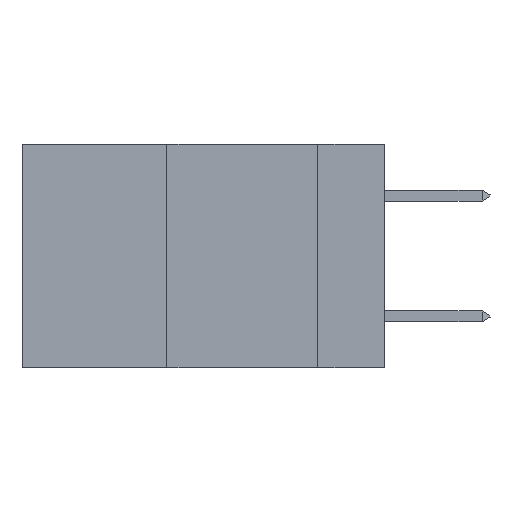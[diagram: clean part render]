
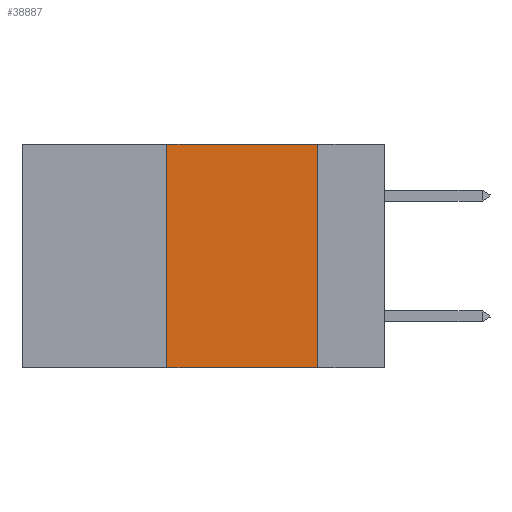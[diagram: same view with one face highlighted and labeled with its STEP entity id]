
A CAD part, left-side view. The second image highlights one B-rep face of the part: STEP entity #38887.
In plain terms, the highlighted planar face has unit normal (-1, 0, 0).
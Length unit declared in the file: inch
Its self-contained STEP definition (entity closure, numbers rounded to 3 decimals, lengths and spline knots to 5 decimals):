
#25 = LINE ( 'NONE', #26661, #32144 ) ;
#635 = EDGE_CURVE ( 'NONE', #34357, #15904, #16948, .T. ) ;
#901 = AXIS2_PLACEMENT_3D ( 'NONE', #5681, #37082, #11699 ) ;
#2297 = FACE_OUTER_BOUND ( 'NONE', #4940, .T. ) ;
#3083 = DIRECTION ( 'NONE',  ( 0., 0., 1. ) ) ;
#4938 = ORIENTED_EDGE ( 'NONE', *, *, #16117, .F. ) ;
#4940 = EDGE_LOOP ( 'NONE', ( #39831, #4938, #22129, #20218 ) ) ;
#5237 = LINE ( 'NONE', #14652, #22766 ) ;
#5681 = CARTESIAN_POINT ( 'NONE',  ( 0., 0.6, 0. ) ) ;
#6089 = CARTESIAN_POINT ( 'NONE',  ( 0., 0.36, 0. ) ) ;
#7696 = CARTESIAN_POINT ( 'NONE',  ( 0., 0.11, -0.37 ) ) ;
#11177 = DIRECTION ( 'NONE',  ( 0., 0., -1. ) ) ;
#11699 = DIRECTION ( 'NONE',  ( 0., 0., -1. ) ) ;
#13854 = DIRECTION ( 'NONE',  ( 0., -1., 0. ) ) ;
#14652 = CARTESIAN_POINT ( 'NONE',  ( 0., 0.6, 0. ) ) ;
#15586 = VECTOR ( 'NONE', #3083, 39.37008 ) ;
#15904 = VERTEX_POINT ( 'NONE', #7696 ) ;
#16117 = EDGE_CURVE ( 'NONE', #38313, #36865, #5237, .T. ) ;
#16948 = LINE ( 'NONE', #24063, #29595 ) ;
#17883 = DIRECTION ( 'NONE',  ( 0., -1., 0. ) ) ;
#19986 = CARTESIAN_POINT ( 'NONE',  ( 0., 0.36, 0. ) ) ;
#20218 = ORIENTED_EDGE ( 'NONE', *, *, #635, .T. ) ;
#22129 = ORIENTED_EDGE ( 'NONE', *, *, #32694, .F. ) ;
#22766 = VECTOR ( 'NONE', #17883, 39.37008 ) ;
#24063 = CARTESIAN_POINT ( 'NONE',  ( 0., 0.6, -0.37 ) ) ;
#26237 = LINE ( 'NONE', #6089, #15586 ) ;
#26661 = CARTESIAN_POINT ( 'NONE',  ( 0., 0.11, 0. ) ) ;
#29595 = VECTOR ( 'NONE', #13854, 39.37008 ) ;
#29941 = CARTESIAN_POINT ( 'NONE',  ( 0., 0.11, 0. ) ) ;
#32144 = VECTOR ( 'NONE', #11177, 39.37008 ) ;
#32423 = EDGE_CURVE ( 'NONE', #36865, #15904, #25, .T. ) ;
#32595 = CARTESIAN_POINT ( 'NONE',  ( 0., 0.36, -0.37 ) ) ;
#32694 = EDGE_CURVE ( 'NONE', #34357, #38313, #26237, .T. ) ;
#34357 = VERTEX_POINT ( 'NONE', #32595 ) ;
#36810 = PLANE ( 'NONE',  #901 ) ;
#36865 = VERTEX_POINT ( 'NONE', #29941 ) ;
#37082 = DIRECTION ( 'NONE',  ( 1., 0., 0. ) ) ;
#38313 = VERTEX_POINT ( 'NONE', #19986 ) ;
#38887 = ADVANCED_FACE ( 'NONE', ( #2297 ), #36810, .F. ) ;
#39831 = ORIENTED_EDGE ( 'NONE', *, *, #32423, .F. ) ;
